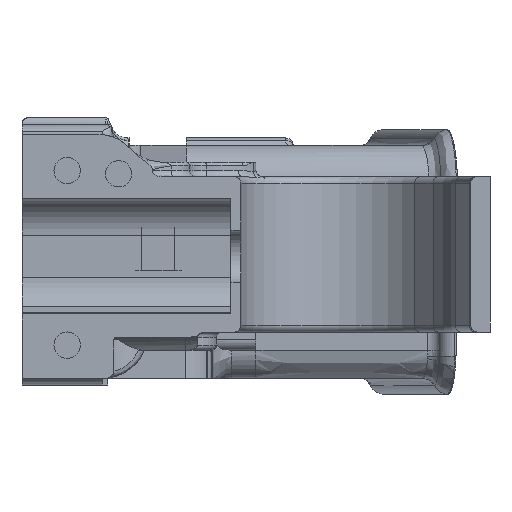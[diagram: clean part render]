
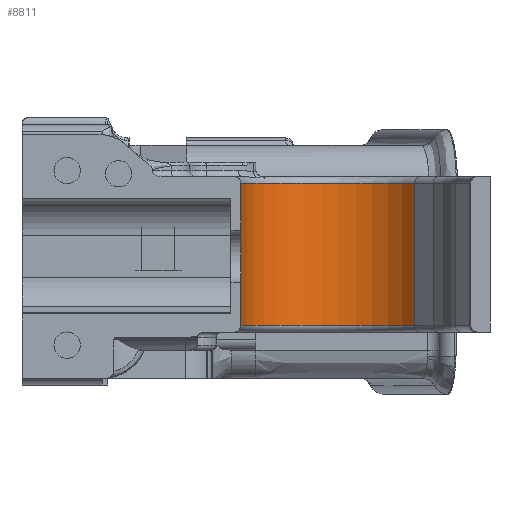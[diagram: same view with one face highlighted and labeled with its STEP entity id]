
A CAD part, left-side view. The second image highlights one B-rep face of the part: STEP entity #8811.
In plain terms, the highlighted cylindrical face has radius 15.081 mm (diameter 30.163 mm), a partial arc.
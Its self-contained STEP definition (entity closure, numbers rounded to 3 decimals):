
#223=CYLINDRICAL_SURFACE('',#9493,15.081);
#543=CIRCLE('',#9486,15.081);
#545=CIRCLE('',#9494,15.081);
#1147=FACE_OUTER_BOUND('',#1664,.T.);
#1664=EDGE_LOOP('',(#7809,#7810,#7811,#7812));
#2271=LINE('',#21081,#2852);
#2296=LINE('',#21850,#2877);
#2852=VECTOR('',#11147,10.);
#2877=VECTOR('',#11312,10.);
#4093=VERTEX_POINT('',#21071);
#4096=VERTEX_POINT('',#21080);
#4144=VERTEX_POINT('',#21792);
#4148=VERTEX_POINT('',#21848);
#5326=EDGE_CURVE('',#4093,#4096,#2271,.T.);
#5414=EDGE_CURVE('',#4144,#4093,#543,.T.);
#5420=EDGE_CURVE('',#4096,#4148,#545,.T.);
#5421=EDGE_CURVE('',#4144,#4148,#2296,.T.);
#7809=ORIENTED_EDGE('',*,*,#5420,.F.);
#7810=ORIENTED_EDGE('',*,*,#5326,.F.);
#7811=ORIENTED_EDGE('',*,*,#5414,.F.);
#7812=ORIENTED_EDGE('',*,*,#5421,.T.);
#8811=ADVANCED_FACE('',(#1147),#223,.F.);
#9486=AXIS2_PLACEMENT_3D('',#21834,#11290,#11291);
#9493=AXIS2_PLACEMENT_3D('',#21847,#11308,#11309);
#9494=AXIS2_PLACEMENT_3D('',#21849,#11310,#11311);
#11147=DIRECTION('',(0.,0.,1.));
#11290=DIRECTION('center_axis',(0.,0.,1.));
#11291=DIRECTION('ref_axis',(0.936,0.351,0.));
#11308=DIRECTION('center_axis',(0.,0.,1.));
#11309=DIRECTION('ref_axis',(0.608,0.794,0.));
#11310=DIRECTION('center_axis',(0.,0.,-1.));
#11311=DIRECTION('ref_axis',(0.936,0.351,0.));
#11312=DIRECTION('',(0.,0.,1.));
#21071=CARTESIAN_POINT('',(-122.149,-26.88,-10.509));
#21080=CARTESIAN_POINT('',(-122.149,-26.88,11.109));
#21081=CARTESIAN_POINT('',(-122.149,-26.88,-11.509));
#21792=CARTESIAN_POINT('',(-112.231,-53.322,-10.509));
#21834=CARTESIAN_POINT('Origin',(-122.149,-41.961,-10.509));
#21847=CARTESIAN_POINT('Origin',(-122.149,-41.961,-11.509));
#21848=CARTESIAN_POINT('',(-112.231,-53.322,11.109));
#21849=CARTESIAN_POINT('Origin',(-122.149,-41.961,11.109));
#21850=CARTESIAN_POINT('',(-112.231,-53.322,-11.509));
